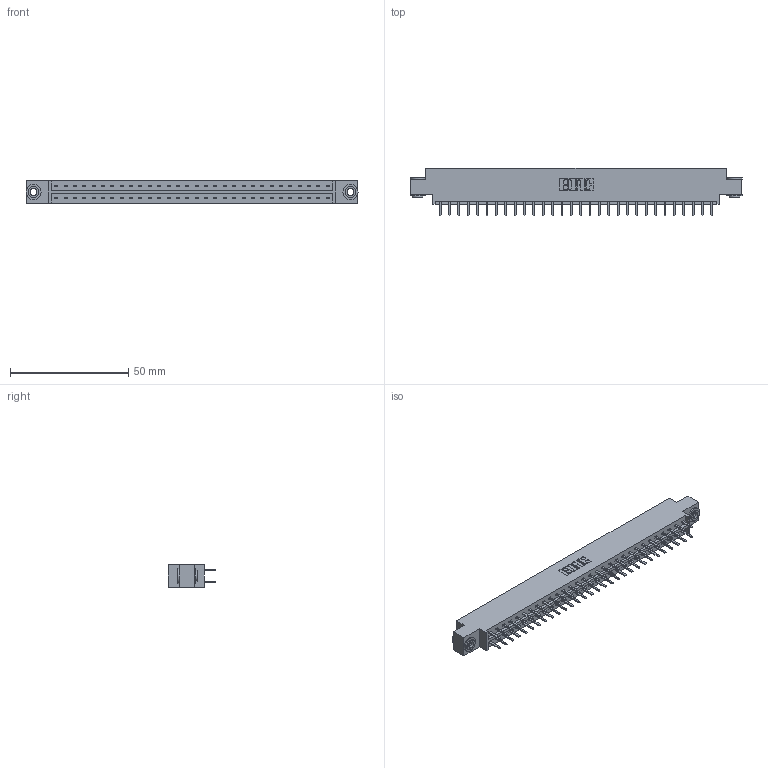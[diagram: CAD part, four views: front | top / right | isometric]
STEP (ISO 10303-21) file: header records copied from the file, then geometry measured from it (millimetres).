
FILE_DESCRIPTION (( 'STEP AP203' ), '1' );
FILE_NAME ('333-060-520-803.STEP', '2018-08-04T06:50:53', ( '' ), ( '' ), 'SwSTEP 2.0', 'SolidWorks 2016', '' );
FILE_SCHEMA (( 'CONFIG_CONTROL_DESIGN' ));
Length unit declared in the file: inch
Products named in the file (4): 333 Part_Offset - .156 Dia - TH; 345-292-001_345-293-120; 345-250-002_345-250-002-102; 333-060-520-803
Assembly tree (63 placements, depth 2):
  333-060-520-803
    333 Part_Offset - .156 Dia - TH
    345-292-001_345-293-120  x60
    345-250-002_345-250-002-102  x2
Bounding box: 140.41 x 20.02 x 9.4 mm (x, y, z)
Volume: 13988.2 mm3; surface area: 16780.4 mm2
Topology: 63 solids, 63 shells, 3516 faces, 10179 edges, 6622 vertices
Faces by surface type: plane 2364, cylinder 1144, cone 8
Entity records: 21748 total; most frequent: CARTESIAN_POINT 3609, ORIENTED_EDGE 3526, DIRECTION 3125, EDGE_CURVE 1763, VECTOR 1607, LINE 1607, VERTEX_POINT 1170, AXIS2_PLACEMENT_3D 759
